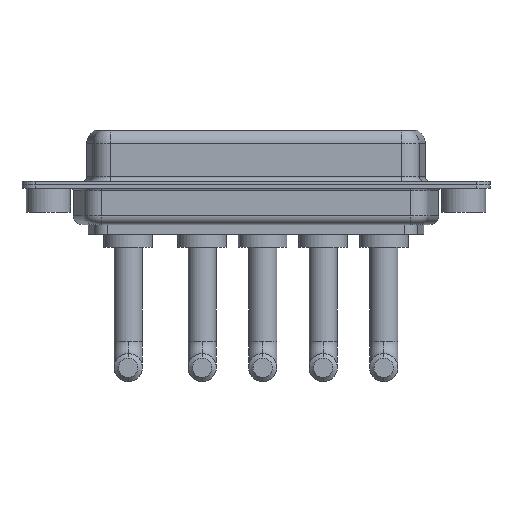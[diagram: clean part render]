
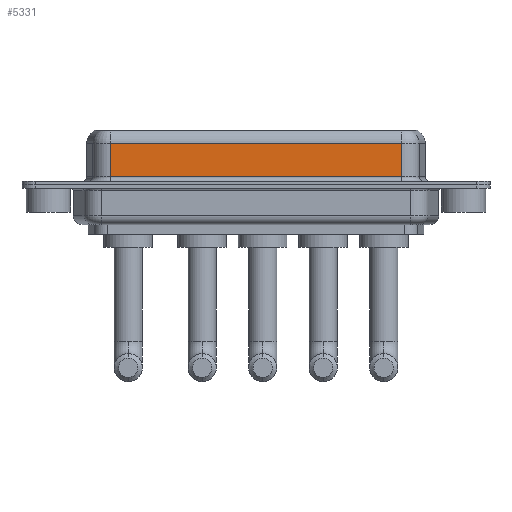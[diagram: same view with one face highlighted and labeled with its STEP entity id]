
A CAD part, front view. The second image highlights one B-rep face of the part: STEP entity #5331.
In plain terms, the highlighted planar face has unit normal (0, -1, 0).
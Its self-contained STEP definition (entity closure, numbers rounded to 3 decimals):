
#111 = PLANE ( 'NONE',  #3181 ) ;
#807 = VERTEX_POINT ( 'NONE', #9796 ) ;
#965 = CARTESIAN_POINT ( 'NONE',  ( 40.037, -3.95, 6.4 ) ) ;
#1245 = EDGE_CURVE ( 'NONE', #807, #11759, #10177, .T. ) ;
#1268 = DIRECTION ( 'NONE',  ( 0., 1., 0. ) ) ;
#1464 = CARTESIAN_POINT ( 'NONE',  ( 40.037, -3.95, 4.65 ) ) ;
#1572 = VECTOR ( 'NONE', #8377, 1000. ) ;
#1606 = DIRECTION ( 'NONE',  ( 1., 0., 0. ) ) ;
#1727 = EDGE_CURVE ( 'NONE', #11759, #4032, #6414, .T. ) ;
#2422 = DIRECTION ( 'NONE',  ( -1., 0., 0. ) ) ;
#3181 = AXIS2_PLACEMENT_3D ( 'NONE', #5949, #1268, #4151 ) ;
#3516 = CARTESIAN_POINT ( 'NONE',  ( 40.037, -3.95, 0.9 ) ) ;
#3726 = EDGE_CURVE ( 'NONE', #5059, #4032, #9696, .T. ) ;
#4032 = VERTEX_POINT ( 'NONE', #3516 ) ;
#4151 = DIRECTION ( 'NONE',  ( 0., 0., 1. ) ) ;
#4349 = ORIENTED_EDGE ( 'NONE', *, *, #1727, .T. ) ;
#4355 = CARTESIAN_POINT ( 'NONE',  ( 40.037, -3.95, 4.65 ) ) ;
#4729 = FACE_OUTER_BOUND ( 'NONE', #5116, .T. ) ;
#5059 = VERTEX_POINT ( 'NONE', #1464 ) ;
#5116 = EDGE_LOOP ( 'NONE', ( #6840, #6197, #8504, #4349 ) ) ;
#5321 = LINE ( 'NONE', #4355, #8932 ) ;
#5331 = ADVANCED_FACE ( 'NONE', ( #4729 ), #111, .F. ) ;
#5710 = CARTESIAN_POINT ( 'NONE',  ( 40.037, -3.95, 0.9 ) ) ;
#5949 = CARTESIAN_POINT ( 'NONE',  ( 40.037, -3.95, 6.4 ) ) ;
#6197 = ORIENTED_EDGE ( 'NONE', *, *, #6974, .T. ) ;
#6414 = LINE ( 'NONE', #5710, #8566 ) ;
#6840 = ORIENTED_EDGE ( 'NONE', *, *, #3726, .F. ) ;
#6974 = EDGE_CURVE ( 'NONE', #5059, #807, #5321, .T. ) ;
#8377 = DIRECTION ( 'NONE',  ( 0., 0., -1. ) ) ;
#8425 = CARTESIAN_POINT ( 'NONE',  ( 7.013, -3.95, 0.9 ) ) ;
#8504 = ORIENTED_EDGE ( 'NONE', *, *, #1245, .T. ) ;
#8566 = VECTOR ( 'NONE', #1606, 1000. ) ;
#8932 = VECTOR ( 'NONE', #2422, 1000. ) ;
#9196 = VECTOR ( 'NONE', #10801, 1000. ) ;
#9217 = CARTESIAN_POINT ( 'NONE',  ( 7.013, -3.95, 6.4 ) ) ;
#9696 = LINE ( 'NONE', #965, #9196 ) ;
#9796 = CARTESIAN_POINT ( 'NONE',  ( 7.013, -3.95, 4.65 ) ) ;
#10177 = LINE ( 'NONE', #9217, #1572 ) ;
#10801 = DIRECTION ( 'NONE',  ( 0., 0., -1. ) ) ;
#11759 = VERTEX_POINT ( 'NONE', #8425 ) ;
